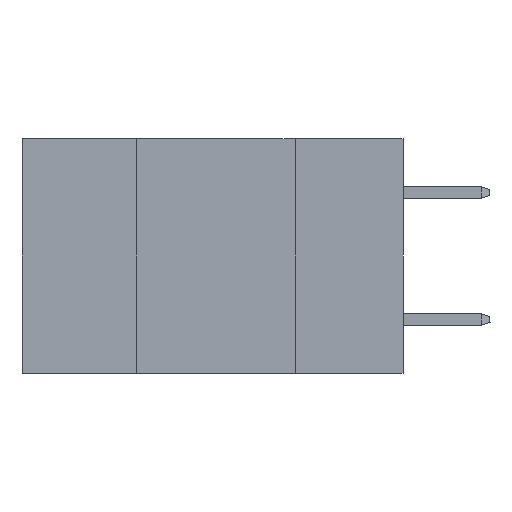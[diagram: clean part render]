
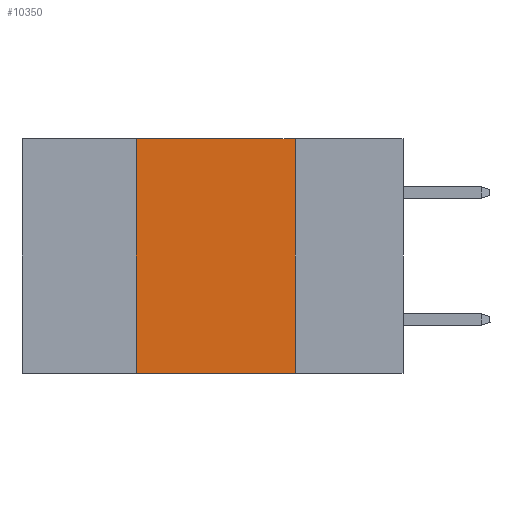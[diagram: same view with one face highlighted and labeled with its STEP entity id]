
A CAD part, left-side view. The second image highlights one B-rep face of the part: STEP entity #10350.
In plain terms, the highlighted planar face has unit normal (-1, 0, 0).
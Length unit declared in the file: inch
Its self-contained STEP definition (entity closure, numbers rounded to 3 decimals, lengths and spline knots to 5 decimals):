
#725 = DIRECTION ( 'NONE',  ( 0., 0., -1. ) ) ;
#1230 = VECTOR ( 'NONE', #7334, 39.37008 ) ;
#1308 = CARTESIAN_POINT ( 'NONE',  ( 0., 0.6, 0. ) ) ;
#1756 = CARTESIAN_POINT ( 'NONE',  ( 0., 0.6, -0.37 ) ) ;
#2175 = ORIENTED_EDGE ( 'NONE', *, *, #7961, .F. ) ;
#4786 = VECTOR ( 'NONE', #6652, 39.37008 ) ;
#5038 = VERTEX_POINT ( 'NONE', #9163 ) ;
#6035 = EDGE_CURVE ( 'NONE', #6381, #6039, #9971, .T. ) ;
#6039 = VERTEX_POINT ( 'NONE', #7078 ) ;
#6381 = VERTEX_POINT ( 'NONE', #13507 ) ;
#6416 = CARTESIAN_POINT ( 'NONE',  ( 0., 0.17, 0. ) ) ;
#6652 = DIRECTION ( 'NONE',  ( 0., 0., 1. ) ) ;
#6716 = EDGE_CURVE ( 'NONE', #5038, #17505, #9090, .T. ) ;
#7078 = CARTESIAN_POINT ( 'NONE',  ( 0., 0.17, -0.37 ) ) ;
#7334 = DIRECTION ( 'NONE',  ( 0., -1., 0. ) ) ;
#7586 = CARTESIAN_POINT ( 'NONE',  ( 0., 0.6, 0. ) ) ;
#7961 = EDGE_CURVE ( 'NONE', #6381, #5038, #8233, .T. ) ;
#8233 = LINE ( 'NONE', #9837, #4786 ) ;
#8939 = ORIENTED_EDGE ( 'NONE', *, *, #6716, .F. ) ;
#9057 = AXIS2_PLACEMENT_3D ( 'NONE', #1308, #14031, #11184 ) ;
#9090 = LINE ( 'NONE', #7586, #12102 ) ;
#9163 = CARTESIAN_POINT ( 'NONE',  ( 0., 0.42, 0. ) ) ;
#9737 = CARTESIAN_POINT ( 'NONE',  ( 0., 0.17, 0. ) ) ;
#9837 = CARTESIAN_POINT ( 'NONE',  ( 0., 0.42, 0. ) ) ;
#9894 = FACE_OUTER_BOUND ( 'NONE', #15358, .T. ) ;
#9971 = LINE ( 'NONE', #1756, #1230 ) ;
#10132 = EDGE_CURVE ( 'NONE', #17505, #6039, #10623, .T. ) ;
#10350 = ADVANCED_FACE ( 'NONE', ( #9894 ), #15225, .F. ) ;
#10623 = LINE ( 'NONE', #6416, #16118 ) ;
#11184 = DIRECTION ( 'NONE',  ( 0., 0., -1. ) ) ;
#12102 = VECTOR ( 'NONE', #17298, 39.37008 ) ;
#13507 = CARTESIAN_POINT ( 'NONE',  ( 0., 0.42, -0.37 ) ) ;
#14031 = DIRECTION ( 'NONE',  ( 1., 0., 0. ) ) ;
#14074 = ORIENTED_EDGE ( 'NONE', *, *, #6035, .T. ) ;
#14912 = ORIENTED_EDGE ( 'NONE', *, *, #10132, .F. ) ;
#15225 = PLANE ( 'NONE',  #9057 ) ;
#15358 = EDGE_LOOP ( 'NONE', ( #14912, #8939, #2175, #14074 ) ) ;
#16118 = VECTOR ( 'NONE', #725, 39.37008 ) ;
#17298 = DIRECTION ( 'NONE',  ( 0., -1., 0. ) ) ;
#17505 = VERTEX_POINT ( 'NONE', #9737 ) ;
